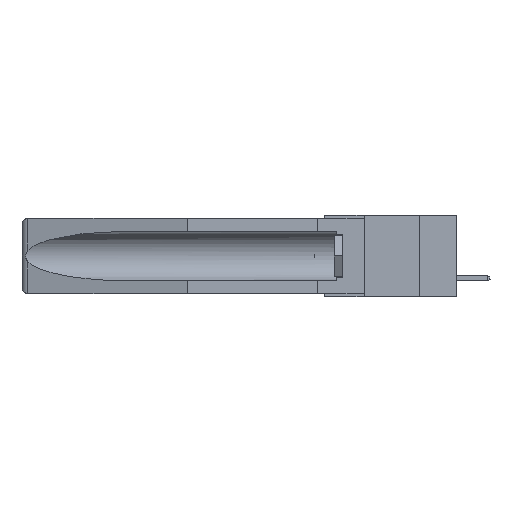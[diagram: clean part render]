
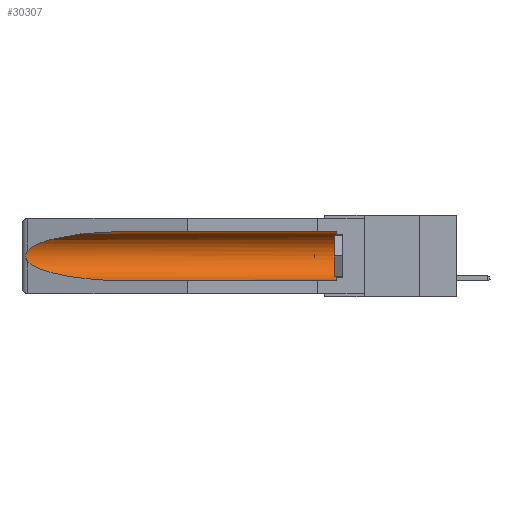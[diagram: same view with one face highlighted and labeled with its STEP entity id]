
A CAD part, left-side view. The second image highlights one B-rep face of the part: STEP entity #30307.
In plain terms, the highlighted cylindrical face has radius 2.857 mm (diameter 5.715 mm), a partial arc.
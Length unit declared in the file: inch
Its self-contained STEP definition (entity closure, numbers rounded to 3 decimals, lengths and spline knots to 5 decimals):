
#215 = CARTESIAN_POINT ( 'NONE',  ( 0.26537, 1.52718, -0.19328 ) ) ;
#745 = EDGE_CURVE ( 'NONE', #5895, #3441, #31722, .T. ) ;
#2201 = DIRECTION ( 'NONE',  ( 0., 0., 1. ) ) ;
#2703 =( BOUNDED_CURVE ( )  B_SPLINE_CURVE ( 3, ( #6854, #33487, #23119, #17901 ),
 .UNSPECIFIED., .F., .F. ) 
 B_SPLINE_CURVE_WITH_KNOTS ( ( 4, 4 ),
 ( 4.71239, 6.08839 ),
 .UNSPECIFIED. ) 
 CURVE ( )  GEOMETRIC_REPRESENTATION_ITEM ( )  RATIONAL_B_SPLINE_CURVE ( ( 1., 0.848, 0.848, 1. ) ) 
 REPRESENTATION_ITEM ( '' )  );
#2749 = CARTESIAN_POINT ( 'NONE',  ( 0.26597, 1.52961, -0.15275 ) ) ;
#2777 = CARTESIAN_POINT ( 'NONE',  ( 0.155, -0.30754, -0.284 ) ) ;
#3110 = FACE_OUTER_BOUND ( 'NONE', #16377, .T. ) ;
#3220 = VERTEX_POINT ( 'NONE', #6392 ) ;
#3441 = VERTEX_POINT ( 'NONE', #23682 ) ;
#3819 = DIRECTION ( 'NONE',  ( 0., 1., 0. ) ) ;
#4320 = VERTEX_POINT ( 'NONE', #4543 ) ;
#4543 = CARTESIAN_POINT ( 'NONE',  ( 0.155, 0.126, -0.059 ) ) ;
#5345 = CARTESIAN_POINT ( 'NONE',  ( 0.26655, 1.53094, -0.18657 ) ) ;
#5540 = EDGE_CURVE ( 'NONE', #3220, #6301, #14059, .T. ) ;
#5895 = VERTEX_POINT ( 'NONE', #24306 ) ;
#6301 = VERTEX_POINT ( 'NONE', #17977 ) ;
#6392 = CARTESIAN_POINT ( 'NONE',  ( 0.155, 0.126, -0.284 ) ) ;
#6854 = CARTESIAN_POINT ( 'NONE',  ( 0.155, 1.07973, -0.059 ) ) ;
#7628 = DIRECTION ( 'NONE',  ( 0., -1., 0. ) ) ;
#7760 = CARTESIAN_POINT ( 'NONE',  ( 0.2673, 1.5327, -0.16383 ) ) ;
#7761 = CARTESIAN_POINT ( 'NONE',  ( 0.155, -0.30754, -0.1715 ) ) ;
#8746 = CARTESIAN_POINT ( 'NONE',  ( 0.26537, 1.52718, -0.19328 ) ) ;
#8963 = CARTESIAN_POINT ( 'NONE',  ( 0.155, 1.07973, -0.059 ) ) ;
#9969 = CARTESIAN_POINT ( 'NONE',  ( 0.155, 0.126, -0.1715 ) ) ;
#10424 = CARTESIAN_POINT ( 'NONE',  ( 0.2675, 1.53308, -0.16763 ) ) ;
#11219 = CARTESIAN_POINT ( 'NONE',  ( 0.155, 1.07973, -0.284 ) ) ;
#11447 = CARTESIAN_POINT ( 'NONE',  ( 0.21114, 1.30732, -0.284 ) ) ;
#11519 = VECTOR ( 'NONE', #26519, 39.37008 ) ;
#12976 = EDGE_CURVE ( 'NONE', #3220, #4320, #28426, .T. ) ;
#13057 = DIRECTION ( 'NONE',  ( 0., 1., 0. ) ) ;
#13506 = CARTESIAN_POINT ( 'NONE',  ( 0.26654, 1.53092, -0.15636 ) ) ;
#14059 = LINE ( 'NONE', #2777, #11519 ) ;
#14651 = ORIENTED_EDGE ( 'NONE', *, *, #25782, .T. ) ;
#15793 = EDGE_CURVE ( 'NONE', #4320, #21730, #30222, .T. ) ;
#16175 = CARTESIAN_POINT ( 'NONE',  ( 0.26597, 1.5296, -0.19026 ) ) ;
#16377 = EDGE_LOOP ( 'NONE', ( #14651, #31303, #18981, #20181, #28627, #26323 ) ) ;
#16576 = CARTESIAN_POINT ( 'NONE',  ( 0.155, -0.30754, -0.059 ) ) ;
#17901 = CARTESIAN_POINT ( 'NONE',  ( 0.26537, 1.52718, -0.14972 ) ) ;
#17977 = CARTESIAN_POINT ( 'NONE',  ( 0.155, 1.07973, -0.284 ) ) ;
#18310 =( BOUNDED_CURVE ( )  B_SPLINE_CURVE ( 3, ( #8746, #19173, #11447, #11219 ),
 .UNSPECIFIED., .F., .F. ) 
 B_SPLINE_CURVE_WITH_KNOTS ( ( 4, 4 ),
 ( 0.1948, 1.5708 ),
 .UNSPECIFIED. ) 
 CURVE ( )  GEOMETRIC_REPRESENTATION_ITEM ( )  RATIONAL_B_SPLINE_CURVE ( ( 1., 0.848, 0.848, 1. ) ) 
 REPRESENTATION_ITEM ( '' )  );
#18610 = CARTESIAN_POINT ( 'NONE',  ( 0.26537, 1.52718, -0.14972 ) ) ;
#18981 = ORIENTED_EDGE ( 'NONE', *, *, #20969, .T. ) ;
#19001 = VECTOR ( 'NONE', #3819, 39.37008 ) ;
#19173 = CARTESIAN_POINT ( 'NONE',  ( 0.25451, 1.48313, -0.24835 ) ) ;
#20181 = ORIENTED_EDGE ( 'NONE', *, *, #5540, .F. ) ;
#20794 = AXIS2_PLACEMENT_3D ( 'NONE', #9969, #7628, #31162 ) ;
#20969 = EDGE_CURVE ( 'NONE', #3441, #6301, #18310, .T. ) ;
#21244 = CARTESIAN_POINT ( 'NONE',  ( 0.2673, 1.53269, -0.17917 ) ) ;
#21730 = VERTEX_POINT ( 'NONE', #8963 ) ;
#23119 = CARTESIAN_POINT ( 'NONE',  ( 0.25451, 1.48313, -0.09465 ) ) ;
#23682 = CARTESIAN_POINT ( 'NONE',  ( 0.26537, 1.52718, -0.19328 ) ) ;
#24306 = CARTESIAN_POINT ( 'NONE',  ( 0.26537, 1.52718, -0.14972 ) ) ;
#25782 = EDGE_CURVE ( 'NONE', #21730, #5895, #2703, .T. ) ;
#26016 = AXIS2_PLACEMENT_3D ( 'NONE', #7761, #13057, #2201 ) ;
#26323 = ORIENTED_EDGE ( 'NONE', *, *, #15793, .T. ) ;
#26519 = DIRECTION ( 'NONE',  ( 0., 1., 0. ) ) ;
#28426 = CIRCLE ( 'NONE', #20794, 0.1125 ) ;
#28627 = ORIENTED_EDGE ( 'NONE', *, *, #12976, .T. ) ;
#30222 = LINE ( 'NONE', #16576, #19001 ) ;
#30307 = ADVANCED_FACE ( 'NONE', ( #3110 ), #31439, .F. ) ;
#31162 = DIRECTION ( 'NONE',  ( 0., 0., 1. ) ) ;
#31303 = ORIENTED_EDGE ( 'NONE', *, *, #745, .T. ) ;
#31439 = CYLINDRICAL_SURFACE ( 'NONE', #26016, 0.1125 ) ;
#31722 = B_SPLINE_CURVE_WITH_KNOTS ( 'NONE', 3,
 ( #18610, #2749, #13506, #7760, #10424, #32074, #21244, #5345, #16175, #215 ),
 .UNSPECIFIED., .F., .F.,
 ( 4, 2, 2, 2, 4 ),
 ( 0., 0.00029, 0.00058, 0.00087, 0.00117 ),
 .UNSPECIFIED. ) ;
#32074 = CARTESIAN_POINT ( 'NONE',  ( 0.2675, 1.53308, -0.17534 ) ) ;
#33487 = CARTESIAN_POINT ( 'NONE',  ( 0.21114, 1.30732, -0.059 ) ) ;
